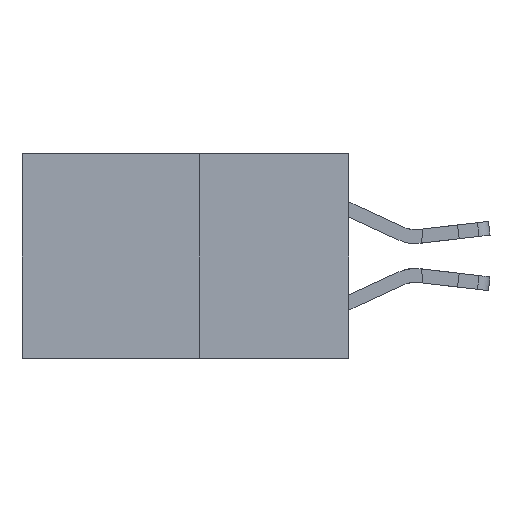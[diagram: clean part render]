
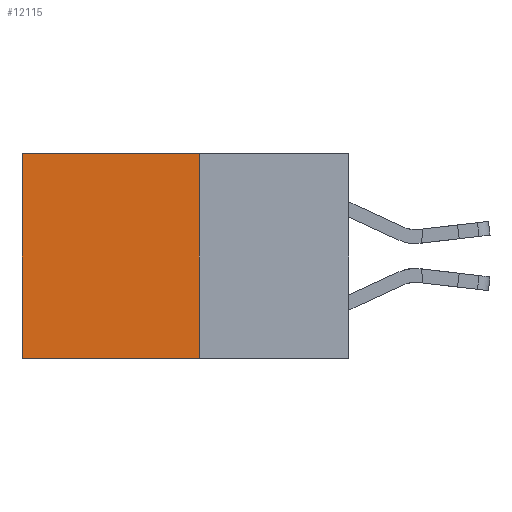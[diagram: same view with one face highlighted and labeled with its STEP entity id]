
A CAD part, left-side view. The second image highlights one B-rep face of the part: STEP entity #12115.
In plain terms, the highlighted planar face has unit normal (-1, 0, 0).
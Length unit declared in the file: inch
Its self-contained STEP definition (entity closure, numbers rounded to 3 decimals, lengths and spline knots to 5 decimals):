
#169 = VECTOR ( 'NONE', #9524, 39.37008 ) ;
#1363 = CARTESIAN_POINT ( 'NONE',  ( 0.277, 0.59, -0.37 ) ) ;
#1939 = DIRECTION ( 'NONE',  ( 0., 1., 0. ) ) ;
#2872 = CARTESIAN_POINT ( 'NONE',  ( 0.277, 0.27, -0.37 ) ) ;
#3656 = CARTESIAN_POINT ( 'NONE',  ( 0.277, 0.27, -0.37 ) ) ;
#3872 = FACE_OUTER_BOUND ( 'NONE', #17434, .T. ) ;
#4174 = VECTOR ( 'NONE', #20326, 39.37008 ) ;
#4884 = DIRECTION ( 'NONE',  ( 0., 0., -1. ) ) ;
#7283 = DIRECTION ( 'NONE',  ( 0., 0., -1. ) ) ;
#7529 = VERTEX_POINT ( 'NONE', #19331 ) ;
#8692 = PLANE ( 'NONE',  #19862 ) ;
#8744 = LINE ( 'NONE', #17617, #13137 ) ;
#9524 = DIRECTION ( 'NONE',  ( 0., 1., 0. ) ) ;
#11615 = CARTESIAN_POINT ( 'NONE',  ( 0.277, 0.27, 0. ) ) ;
#11687 = EDGE_CURVE ( 'NONE', #23556, #24545, #19399, .T. ) ;
#12115 = ADVANCED_FACE ( 'NONE', ( #3872 ), #8692, .F. ) ;
#13137 = VECTOR ( 'NONE', #1939, 39.37008 ) ;
#15876 = ORIENTED_EDGE ( 'NONE', *, *, #11687, .F. ) ;
#16035 = EDGE_CURVE ( 'NONE', #24394, #7529, #21793, .T. ) ;
#16257 = DIRECTION ( 'NONE',  ( 1., 0., 0. ) ) ;
#16671 = VECTOR ( 'NONE', #7283, 39.37008 ) ;
#17434 = EDGE_LOOP ( 'NONE', ( #20579, #18266, #15876, #21993 ) ) ;
#17597 = CARTESIAN_POINT ( 'NONE',  ( 0.277, 0.59, 0. ) ) ;
#17617 = CARTESIAN_POINT ( 'NONE',  ( 0.277, 0.27, 0. ) ) ;
#18266 = ORIENTED_EDGE ( 'NONE', *, *, #24142, .F. ) ;
#18355 = CARTESIAN_POINT ( 'NONE',  ( 0.277, 0.27, -0.37 ) ) ;
#19331 = CARTESIAN_POINT ( 'NONE',  ( 0.277, 0.59, -0.37 ) ) ;
#19399 = LINE ( 'NONE', #18355, #4174 ) ;
#19862 = AXIS2_PLACEMENT_3D ( 'NONE', #2872, #16257, #4884 ) ;
#20326 = DIRECTION ( 'NONE',  ( 0., 0., -1. ) ) ;
#20579 = ORIENTED_EDGE ( 'NONE', *, *, #16035, .T. ) ;
#20632 = LINE ( 'NONE', #3656, #169 ) ;
#21793 = LINE ( 'NONE', #1363, #16671 ) ;
#21796 = CARTESIAN_POINT ( 'NONE',  ( 0.277, 0.27, -0.37 ) ) ;
#21993 = ORIENTED_EDGE ( 'NONE', *, *, #24229, .T. ) ;
#23556 = VERTEX_POINT ( 'NONE', #11615 ) ;
#24142 = EDGE_CURVE ( 'NONE', #24545, #7529, #20632, .T. ) ;
#24229 = EDGE_CURVE ( 'NONE', #23556, #24394, #8744, .T. ) ;
#24394 = VERTEX_POINT ( 'NONE', #17597 ) ;
#24545 = VERTEX_POINT ( 'NONE', #21796 ) ;
